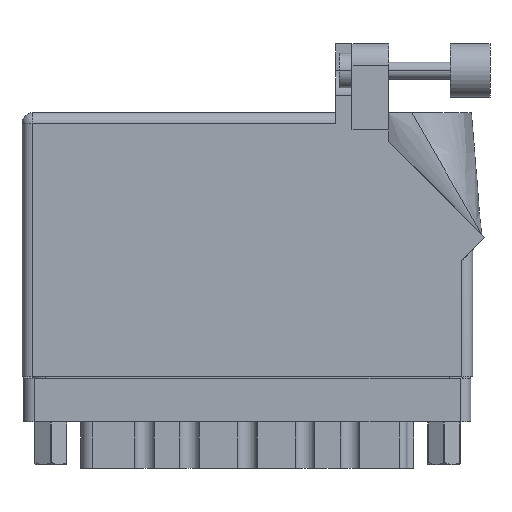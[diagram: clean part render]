
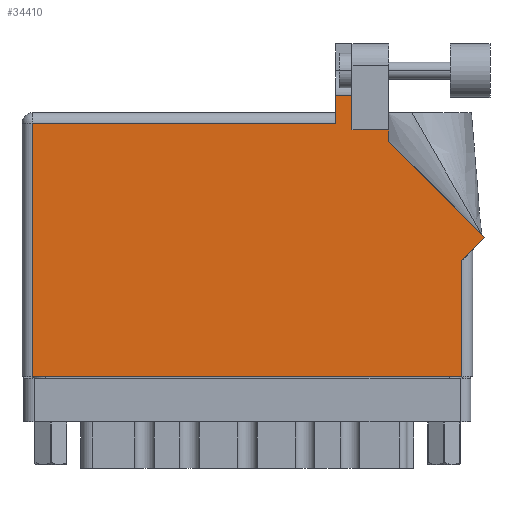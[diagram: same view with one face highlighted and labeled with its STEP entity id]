
A CAD part, front view. The second image highlights one B-rep face of the part: STEP entity #34410.
In plain terms, the highlighted face is planar.
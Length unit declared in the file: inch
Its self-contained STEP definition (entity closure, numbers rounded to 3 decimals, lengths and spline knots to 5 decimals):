
#1758 = LINE ( 'NONE', #8623, #40219 ) ;
#1940 = VECTOR ( 'NONE', #44778, 39.37008 ) ;
#2766 = EDGE_CURVE ( 'NONE', #19717, #61118, #57671, .T. ) ;
#3537 = CARTESIAN_POINT ( 'NONE',  ( 0.062, 1.468, 0. ) ) ;
#3765 = EDGE_CURVE ( 'NONE', #26519, #46065, #62113, .T. ) ;
#6657 = ORIENTED_EDGE ( 'NONE', *, *, #41408, .T. ) ;
#6788 = ORIENTED_EDGE ( 'NONE', *, *, #40670, .T. ) ;
#8417 = VECTOR ( 'NONE', #41727, 39.37008 ) ;
#8623 = CARTESIAN_POINT ( 'NONE',  ( 1.913, 1.43, 0. ) ) ;
#9311 = CARTESIAN_POINT ( 'NONE',  ( 0., 1.53, 0. ) ) ;
#10347 = VERTEX_POINT ( 'NONE', #12436 ) ;
#10582 = DIRECTION ( 'NONE',  ( 1., 0., 0. ) ) ;
#11432 = CARTESIAN_POINT ( 'NONE',  ( 2.68271, 0.80771, 0. ) ) ;
#11632 = CARTESIAN_POINT ( 'NONE',  ( 2.126, 1.43, 0. ) ) ;
#11804 = EDGE_CURVE ( 'NONE', #60959, #12723, #12962, .T. ) ;
#11832 = CARTESIAN_POINT ( 'NONE',  ( 2.55, 0., 0. ) ) ;
#12436 = CARTESIAN_POINT ( 'NONE',  ( 1.913, 1.6315, 0. ) ) ;
#12723 = VERTEX_POINT ( 'NONE', #14197 ) ;
#12962 = LINE ( 'NONE', #62541, #18184 ) ;
#13540 = LINE ( 'NONE', #11632, #18732 ) ;
#13704 = VERTEX_POINT ( 'NONE', #26262 ) ;
#14197 = CARTESIAN_POINT ( 'NONE',  ( 2.55, 0.675, 0. ) ) ;
#14302 = DIRECTION ( 'NONE',  ( 0., 1., 0. ) ) ;
#14492 = DIRECTION ( 'NONE',  ( 0., 1., 0. ) ) ;
#14691 = EDGE_CURVE ( 'NONE', #17259, #13704, #54817, .T. ) ;
#15754 = EDGE_CURVE ( 'NONE', #59924, #10347, #1758, .T. ) ;
#16026 = VERTEX_POINT ( 'NONE', #22797 ) ;
#17259 = VERTEX_POINT ( 'NONE', #59348 ) ;
#17399 = CARTESIAN_POINT ( 'NONE',  ( 2.68271, 0.80771, 0. ) ) ;
#18184 = VECTOR ( 'NONE', #14302, 39.37008 ) ;
#18732 = VECTOR ( 'NONE', #31568, 39.37008 ) ;
#18916 = DIRECTION ( 'NONE',  ( 0., 0., -1. ) ) ;
#19222 = EDGE_CURVE ( 'NONE', #13704, #19717, #38013, .T. ) ;
#19717 = VERTEX_POINT ( 'NONE', #3537 ) ;
#20540 = ORIENTED_EDGE ( 'NONE', *, *, #11804, .T. ) ;
#22797 = CARTESIAN_POINT ( 'NONE',  ( 2.126, 1.43, 0. ) ) ;
#24838 = ORIENTED_EDGE ( 'NONE', *, *, #19222, .T. ) ;
#25578 = VECTOR ( 'NONE', #56873, 39.37008 ) ;
#26040 = ORIENTED_EDGE ( 'NONE', *, *, #2766, .T. ) ;
#26262 = CARTESIAN_POINT ( 'NONE',  ( 1.819, 1.468, 0. ) ) ;
#26519 = VERTEX_POINT ( 'NONE', #11432 ) ;
#26586 = DIRECTION ( 'NONE',  ( -1., 0., 0. ) ) ;
#26748 = VECTOR ( 'NONE', #54928, 39.37008 ) ;
#27141 = ORIENTED_EDGE ( 'NONE', *, *, #3765, .T. ) ;
#27761 = ORIENTED_EDGE ( 'NONE', *, *, #33267, .T. ) ;
#28275 = EDGE_CURVE ( 'NONE', #46065, #16026, #35336, .T. ) ;
#29214 = VECTOR ( 'NONE', #10582, 39.37008 ) ;
#31568 = DIRECTION ( 'NONE',  ( -1., 0., 0. ) ) ;
#33267 = EDGE_CURVE ( 'NONE', #10347, #17259, #40051, .T. ) ;
#34410 = ADVANCED_FACE ( 'NONE', ( #61971 ), #47940, .F. ) ;
#34884 = ORIENTED_EDGE ( 'NONE', *, *, #28275, .T. ) ;
#35336 = LINE ( 'NONE', #53383, #46777 ) ;
#36678 = ORIENTED_EDGE ( 'NONE', *, *, #15754, .T. ) ;
#37814 = CARTESIAN_POINT ( 'NONE',  ( 2.24377, 1.6315, 0. ) ) ;
#38013 = LINE ( 'NONE', #55655, #47154 ) ;
#39183 = ORIENTED_EDGE ( 'NONE', *, *, #14691, .T. ) ;
#40051 = LINE ( 'NONE', #37814, #25578 ) ;
#40219 = VECTOR ( 'NONE', #52340, 39.37008 ) ;
#40311 = CARTESIAN_POINT ( 'NONE',  ( 2.612, 0.737, 0. ) ) ;
#40670 = EDGE_CURVE ( 'NONE', #12723, #26519, #56388, .T. ) ;
#41408 = EDGE_CURVE ( 'NONE', #61118, #60959, #55012, .T. ) ;
#41727 = DIRECTION ( 'NONE',  ( -0.707, 0.707, 0. ) ) ;
#43878 = AXIS2_PLACEMENT_3D ( 'NONE', #9311, #18916, #47723 ) ;
#44778 = DIRECTION ( 'NONE',  ( 0.707, 0.707, 0. ) ) ;
#45299 = ORIENTED_EDGE ( 'NONE', *, *, #48277, .T. ) ;
#45513 = DIRECTION ( 'NONE',  ( 0., -1., 0. ) ) ;
#46065 = VERTEX_POINT ( 'NONE', #49694 ) ;
#46777 = VECTOR ( 'NONE', #14492, 39.37008 ) ;
#47067 = VECTOR ( 'NONE', #45513, 39.37008 ) ;
#47154 = VECTOR ( 'NONE', #26586, 39.37008 ) ;
#47723 = DIRECTION ( 'NONE',  ( -1., 0., 0. ) ) ;
#47940 = PLANE ( 'NONE',  #43878 ) ;
#48277 = EDGE_CURVE ( 'NONE', #16026, #59924, #13540, .T. ) ;
#49694 = CARTESIAN_POINT ( 'NONE',  ( 2.126, 1.36442, 0. ) ) ;
#50610 = CARTESIAN_POINT ( 'NONE',  ( 0.062, 0., 0. ) ) ;
#51351 = CARTESIAN_POINT ( 'NONE',  ( 0.062, 0., 0. ) ) ;
#52340 = DIRECTION ( 'NONE',  ( 0., 1., 0. ) ) ;
#53383 = CARTESIAN_POINT ( 'NONE',  ( 2.126, 1.36442, 0. ) ) ;
#54112 = CARTESIAN_POINT ( 'NONE',  ( 0., 0., 0. ) ) ;
#54817 = LINE ( 'NONE', #56406, #26748 ) ;
#54928 = DIRECTION ( 'NONE',  ( 0., -1., 0. ) ) ;
#55012 = LINE ( 'NONE', #54112, #29214 ) ;
#55655 = CARTESIAN_POINT ( 'NONE',  ( 0., 1.468, 0. ) ) ;
#56006 = EDGE_LOOP ( 'NONE', ( #36678, #27761, #39183, #24838, #26040, #6657, #20540, #6788, #27141, #34884, #45299 ) ) ;
#56388 = LINE ( 'NONE', #40311, #1940 ) ;
#56406 = CARTESIAN_POINT ( 'NONE',  ( 1.819, 1.53, 0. ) ) ;
#56873 = DIRECTION ( 'NONE',  ( -1., 0., 0. ) ) ;
#57671 = LINE ( 'NONE', #50610, #47067 ) ;
#59348 = CARTESIAN_POINT ( 'NONE',  ( 1.819, 1.6315, 0. ) ) ;
#59924 = VERTEX_POINT ( 'NONE', #61430 ) ;
#60959 = VERTEX_POINT ( 'NONE', #11832 ) ;
#61118 = VERTEX_POINT ( 'NONE', #51351 ) ;
#61430 = CARTESIAN_POINT ( 'NONE',  ( 1.913, 1.43, 0. ) ) ;
#61971 = FACE_OUTER_BOUND ( 'NONE', #56006, .T. ) ;
#62113 = LINE ( 'NONE', #17399, #8417 ) ;
#62541 = CARTESIAN_POINT ( 'NONE',  ( 2.55, 0.737, 0. ) ) ;
